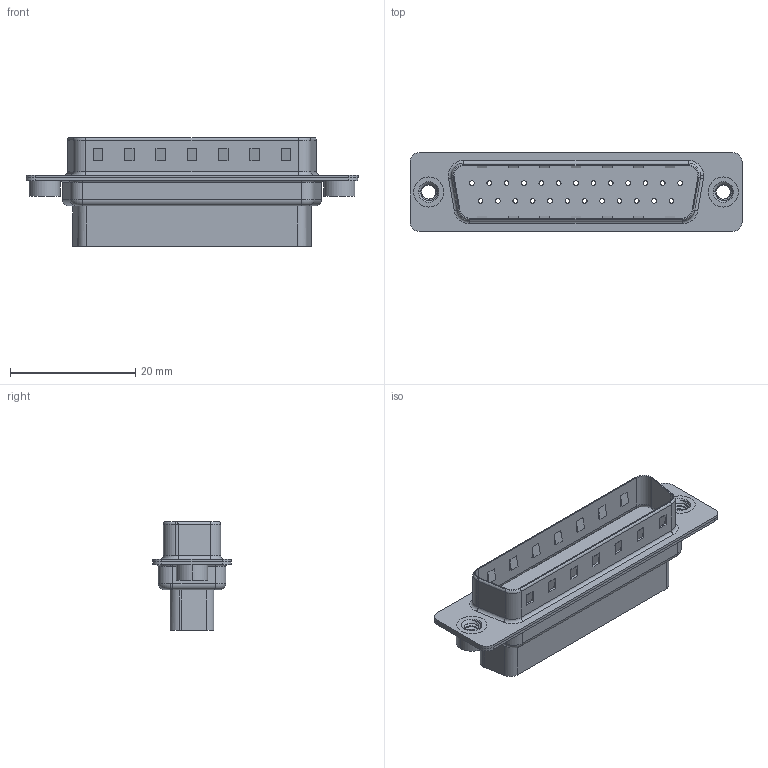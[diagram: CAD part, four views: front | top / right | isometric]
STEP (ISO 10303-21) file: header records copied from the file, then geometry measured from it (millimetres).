
FILE_DESCRIPTION (( 'STEP AP203' ), '1' );
FILE_NAME ('627-025-010-242.STEP', '2020-07-15T20:39:09', ( '' ), ( '' ), 'SwSTEP 2.0', 'SolidWorks 2020', '' );
FILE_SCHEMA (( 'CONFIG_CONTROL_DESIGN' ));
Length unit declared in the file: millimetre
Products named in the file (5): 627-025-010-242; 627 Housing_25 HP; 627 Shell Rear_25 Contacts; 627 4-40 Threaded Rivet; 627 Shell Front_25 Contacts
Assembly tree (5 placements, depth 2):
  627-025-010-242
    627 Housing_25 HP
    627 Shell Front_25 Contacts
    627 Shell Rear_25 Contacts
    627 4-40 Threaded Rivet  x2
Bounding box: 53 x 12.6 x 17.4 mm (x, y, z)
Volume: 3501.2 mm3; surface area: 6608.2 mm2
Topology: 5 solids, 5 shells, 572 faces, 1397 edges, 896 vertices
Faces by surface type: cylinder 285, plane 221, torus 50, cone 10, bspline 6
Entity records: 18134 total; most frequent: CARTESIAN_POINT 4238, DIRECTION 2956, ORIENTED_EDGE 2642, EDGE_CURVE 1321, AXIS2_PLACEMENT_3D 1134, VERTEX_POINT 847, EDGE_LOOP 692, VECTOR 688
